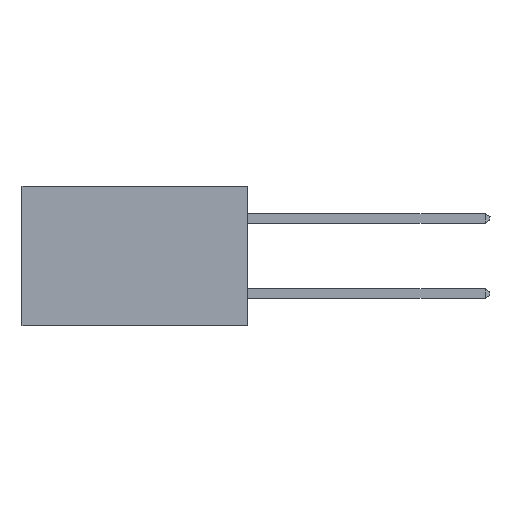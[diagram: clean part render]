
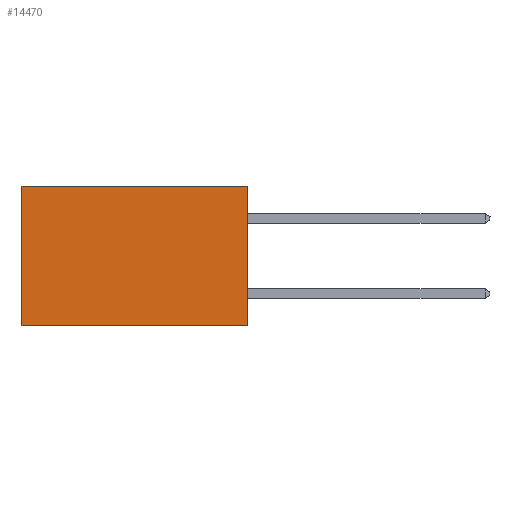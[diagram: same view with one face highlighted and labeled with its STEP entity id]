
A CAD part, left-side view. The second image highlights one B-rep face of the part: STEP entity #14470.
In plain terms, the highlighted planar face has unit normal (-1, 0, 0).
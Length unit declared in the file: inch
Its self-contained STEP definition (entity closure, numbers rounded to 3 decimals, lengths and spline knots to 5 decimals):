
#44 = VECTOR ( 'NONE', #3359, 39.37008 ) ;
#220 = DIRECTION ( 'NONE',  ( 0., 0., -1. ) ) ;
#1175 = CARTESIAN_POINT ( 'NONE',  ( 0.298, 0., -0.37 ) ) ;
#1306 = VECTOR ( 'NONE', #23648, 39.37008 ) ;
#1967 = EDGE_CURVE ( 'NONE', #13947, #5163, #21217, .T. ) ;
#2200 = FACE_OUTER_BOUND ( 'NONE', #14427, .T. ) ;
#2883 = LINE ( 'NONE', #3550, #44 ) ;
#3359 = DIRECTION ( 'NONE',  ( 0., 1., 0. ) ) ;
#3550 = CARTESIAN_POINT ( 'NONE',  ( 0.298, 0., 0. ) ) ;
#5163 = VERTEX_POINT ( 'NONE', #6488 ) ;
#5620 = ORIENTED_EDGE ( 'NONE', *, *, #27939, .T. ) ;
#5680 = CARTESIAN_POINT ( 'NONE',  ( 0.298, 0., 0. ) ) ;
#6488 = CARTESIAN_POINT ( 'NONE',  ( 0.298, 0.6, -0.37 ) ) ;
#6584 = CARTESIAN_POINT ( 'NONE',  ( 0.298, 0., 0. ) ) ;
#8953 = EDGE_CURVE ( 'NONE', #14458, #5163, #28298, .T. ) ;
#9007 = CARTESIAN_POINT ( 'NONE',  ( 0.298, 0., -0.37 ) ) ;
#11260 = CARTESIAN_POINT ( 'NONE',  ( 0.298, 0., 0. ) ) ;
#11632 = PLANE ( 'NONE',  #14257 ) ;
#12498 = VECTOR ( 'NONE', #22469, 39.37008 ) ;
#13947 = VERTEX_POINT ( 'NONE', #18884 ) ;
#14257 = AXIS2_PLACEMENT_3D ( 'NONE', #11260, #27308, #220 ) ;
#14427 = EDGE_LOOP ( 'NONE', ( #14806, #26764, #15780, #5620 ) ) ;
#14458 = VERTEX_POINT ( 'NONE', #9007 ) ;
#14470 = ADVANCED_FACE ( 'NONE', ( #2200 ), #11632, .F. ) ;
#14806 = ORIENTED_EDGE ( 'NONE', *, *, #1967, .T. ) ;
#15780 = ORIENTED_EDGE ( 'NONE', *, *, #18587, .F. ) ;
#18587 = EDGE_CURVE ( 'NONE', #28937, #14458, #23393, .T. ) ;
#18884 = CARTESIAN_POINT ( 'NONE',  ( 0.298, 0.6, 0. ) ) ;
#21217 = LINE ( 'NONE', #25420, #22264 ) ;
#22264 = VECTOR ( 'NONE', #25230, 39.37008 ) ;
#22469 = DIRECTION ( 'NONE',  ( 0., 0., -1. ) ) ;
#23393 = LINE ( 'NONE', #6584, #12498 ) ;
#23648 = DIRECTION ( 'NONE',  ( 0., 1., 0. ) ) ;
#25230 = DIRECTION ( 'NONE',  ( 0., 0., -1. ) ) ;
#25420 = CARTESIAN_POINT ( 'NONE',  ( 0.298, 0.6, 0. ) ) ;
#26764 = ORIENTED_EDGE ( 'NONE', *, *, #8953, .F. ) ;
#27308 = DIRECTION ( 'NONE',  ( 1., 0., 0. ) ) ;
#27939 = EDGE_CURVE ( 'NONE', #28937, #13947, #2883, .T. ) ;
#28298 = LINE ( 'NONE', #1175, #1306 ) ;
#28937 = VERTEX_POINT ( 'NONE', #5680 ) ;
